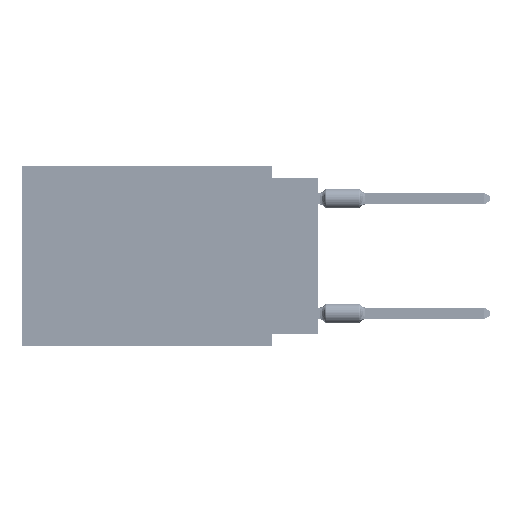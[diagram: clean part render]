
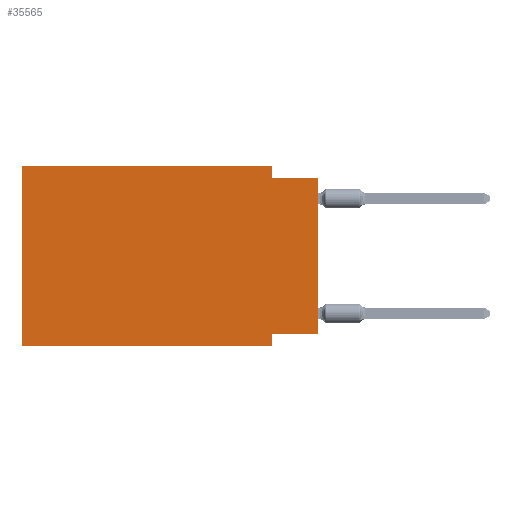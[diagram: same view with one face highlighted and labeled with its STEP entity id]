
A CAD part, left-side view. The second image highlights one B-rep face of the part: STEP entity #35565.
In plain terms, the highlighted planar face has unit normal (-1, 0, 0).
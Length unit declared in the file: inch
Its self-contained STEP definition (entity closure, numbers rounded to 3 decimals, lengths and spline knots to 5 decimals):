
#1904 = CARTESIAN_POINT ( 'NONE',  ( 0., 0.1, -0.39 ) ) ;
#2833 = CARTESIAN_POINT ( 'NONE',  ( 0., 0., -0.365 ) ) ;
#3156 = VERTEX_POINT ( 'NONE', #5190 ) ;
#3469 = CARTESIAN_POINT ( 'NONE',  ( 0., 0., -0.025 ) ) ;
#4053 = CARTESIAN_POINT ( 'NONE',  ( 0., 0., 0. ) ) ;
#4354 = VERTEX_POINT ( 'NONE', #66944 ) ;
#5190 = CARTESIAN_POINT ( 'NONE',  ( 0., 0.645, 0. ) ) ;
#5623 = ORIENTED_EDGE ( 'NONE', *, *, #45518, .F. ) ;
#5919 = CARTESIAN_POINT ( 'NONE',  ( 0., 0.645, -0.39 ) ) ;
#6066 = ORIENTED_EDGE ( 'NONE', *, *, #31475, .F. ) ;
#7142 = EDGE_CURVE ( 'NONE', #39165, #61272, #35261, .T. ) ;
#8765 = EDGE_CURVE ( 'NONE', #4354, #34012, #15759, .T. ) ;
#10723 = ORIENTED_EDGE ( 'NONE', *, *, #8765, .F. ) ;
#10883 = DIRECTION ( 'NONE',  ( 0., 0., -1. ) ) ;
#12014 = VECTOR ( 'NONE', #60771, 39.37008 ) ;
#12096 = ORIENTED_EDGE ( 'NONE', *, *, #67003, .F. ) ;
#13126 = VECTOR ( 'NONE', #18384, 39.37008 ) ;
#13507 = AXIS2_PLACEMENT_3D ( 'NONE', #53943, #16233, #64090 ) ;
#14255 = EDGE_CURVE ( 'NONE', #67404, #57799, #68098, .T. ) ;
#14601 = ORIENTED_EDGE ( 'NONE', *, *, #7142, .F. ) ;
#15118 = CARTESIAN_POINT ( 'NONE',  ( 0., 0.645, 0. ) ) ;
#15759 = LINE ( 'NONE', #31140, #17738 ) ;
#16233 = DIRECTION ( 'NONE',  ( 1., 0., 0. ) ) ;
#17738 = VECTOR ( 'NONE', #10883, 39.37008 ) ;
#17936 = VECTOR ( 'NONE', #52244, 39.37008 ) ;
#18384 = DIRECTION ( 'NONE',  ( 0., 0., 1. ) ) ;
#18913 = EDGE_LOOP ( 'NONE', ( #36503, #5623, #10723, #47735, #6066, #47145, #12096, #14601 ) ) ;
#19540 = DIRECTION ( 'NONE',  ( 0., -1., 0. ) ) ;
#21671 = VECTOR ( 'NONE', #19540, 39.37008 ) ;
#23750 = LINE ( 'NONE', #3469, #21671 ) ;
#28461 = DIRECTION ( 'NONE',  ( 0., 0., -1. ) ) ;
#31137 = CARTESIAN_POINT ( 'NONE',  ( 0., 0., -0.025 ) ) ;
#31140 = CARTESIAN_POINT ( 'NONE',  ( 0., 0.1, 0. ) ) ;
#31475 = EDGE_CURVE ( 'NONE', #67404, #3156, #34453, .T. ) ;
#32651 = LINE ( 'NONE', #39272, #40803 ) ;
#34012 = VERTEX_POINT ( 'NONE', #61571 ) ;
#34453 = LINE ( 'NONE', #44598, #13126 ) ;
#35079 = VECTOR ( 'NONE', #68806, 39.37008 ) ;
#35261 = LINE ( 'NONE', #44710, #12014 ) ;
#35489 = EDGE_CURVE ( 'NONE', #39165, #68894, #58158, .T. ) ;
#35565 = ADVANCED_FACE ( 'NONE', ( #41755 ), #63062, .F. ) ;
#36503 = ORIENTED_EDGE ( 'NONE', *, *, #35489, .T. ) ;
#37105 = LINE ( 'NONE', #15118, #47552 ) ;
#37836 = CARTESIAN_POINT ( 'NONE',  ( 0., 0.645, -0.39 ) ) ;
#39165 = VERTEX_POINT ( 'NONE', #2833 ) ;
#39272 = CARTESIAN_POINT ( 'NONE',  ( 0., 0.1, -0.39 ) ) ;
#40803 = VECTOR ( 'NONE', #28461, 39.37008 ) ;
#41755 = FACE_OUTER_BOUND ( 'NONE', #18913, .T. ) ;
#44598 = CARTESIAN_POINT ( 'NONE',  ( 0., 0.645, 0. ) ) ;
#44710 = CARTESIAN_POINT ( 'NONE',  ( 0., 0., -0.365 ) ) ;
#45518 = EDGE_CURVE ( 'NONE', #34012, #68894, #23750, .T. ) ;
#47145 = ORIENTED_EDGE ( 'NONE', *, *, #14255, .T. ) ;
#47552 = VECTOR ( 'NONE', #57369, 39.37008 ) ;
#47735 = ORIENTED_EDGE ( 'NONE', *, *, #49406, .F. ) ;
#49406 = EDGE_CURVE ( 'NONE', #3156, #4354, #37105, .T. ) ;
#52244 = DIRECTION ( 'NONE',  ( 0., 0., 1. ) ) ;
#53943 = CARTESIAN_POINT ( 'NONE',  ( 0., 0.645, 0. ) ) ;
#57369 = DIRECTION ( 'NONE',  ( 0., -1., 0. ) ) ;
#57799 = VERTEX_POINT ( 'NONE', #1904 ) ;
#58158 = LINE ( 'NONE', #4053, #17936 ) ;
#60771 = DIRECTION ( 'NONE',  ( 0., 1., 0. ) ) ;
#61272 = VERTEX_POINT ( 'NONE', #61348 ) ;
#61348 = CARTESIAN_POINT ( 'NONE',  ( 0., 0.1, -0.365 ) ) ;
#61571 = CARTESIAN_POINT ( 'NONE',  ( 0., 0.1, -0.025 ) ) ;
#63062 = PLANE ( 'NONE',  #13507 ) ;
#64090 = DIRECTION ( 'NONE',  ( 0., 0., -1. ) ) ;
#66944 = CARTESIAN_POINT ( 'NONE',  ( 0., 0.1, 0. ) ) ;
#67003 = EDGE_CURVE ( 'NONE', #61272, #57799, #32651, .T. ) ;
#67404 = VERTEX_POINT ( 'NONE', #37836 ) ;
#68098 = LINE ( 'NONE', #5919, #35079 ) ;
#68806 = DIRECTION ( 'NONE',  ( 0., -1., 0. ) ) ;
#68894 = VERTEX_POINT ( 'NONE', #31137 ) ;
